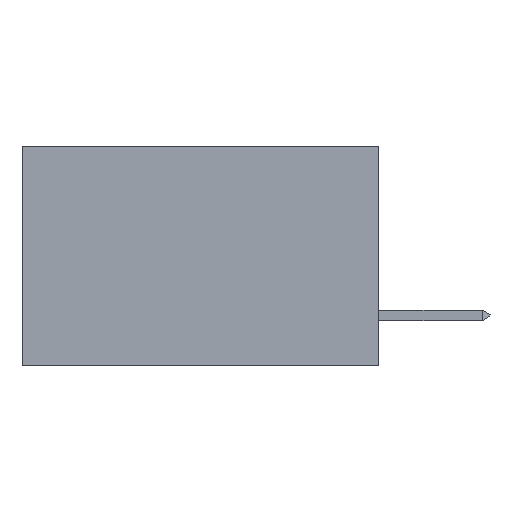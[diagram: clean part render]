
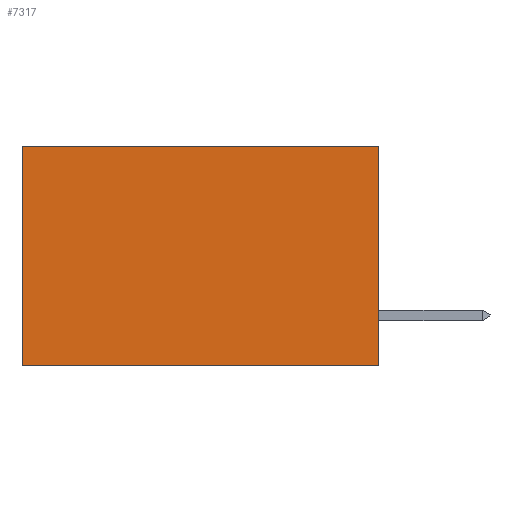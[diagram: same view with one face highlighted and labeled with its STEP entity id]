
A CAD part, left-side view. The second image highlights one B-rep face of the part: STEP entity #7317.
In plain terms, the highlighted planar face has unit normal (-1, 0, 0).
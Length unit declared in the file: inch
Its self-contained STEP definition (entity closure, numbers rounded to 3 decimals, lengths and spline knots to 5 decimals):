
#1004 = EDGE_CURVE ( 'NONE', #13466, #10811, #15204, .T. ) ;
#1601 = ORIENTED_EDGE ( 'NONE', *, *, #4666, .F. ) ;
#1602 = LINE ( 'NONE', #13977, #9259 ) ;
#2469 = LINE ( 'NONE', #5421, #9478 ) ;
#2508 = CARTESIAN_POINT ( 'NONE',  ( 0.298, 0.6, 0. ) ) ;
#3609 = PLANE ( 'NONE',  #8232 ) ;
#3677 = DIRECTION ( 'NONE',  ( 1., 0., 0. ) ) ;
#4666 = EDGE_CURVE ( 'NONE', #5327, #4895, #8896, .T. ) ;
#4877 = VECTOR ( 'NONE', #11938, 39.37008 ) ;
#4895 = VERTEX_POINT ( 'NONE', #14901 ) ;
#5012 = CARTESIAN_POINT ( 'NONE',  ( 0.298, 0., 0. ) ) ;
#5327 = VERTEX_POINT ( 'NONE', #17194 ) ;
#5421 = CARTESIAN_POINT ( 'NONE',  ( 0.298, 0., -0.37 ) ) ;
#7317 = ADVANCED_FACE ( 'NONE', ( #16875 ), #3609, .F. ) ;
#7479 = CARTESIAN_POINT ( 'NONE',  ( 0.298, 0.6, 0. ) ) ;
#7665 = ORIENTED_EDGE ( 'NONE', *, *, #1004, .T. ) ;
#8232 = AXIS2_PLACEMENT_3D ( 'NONE', #5012, #3677, #10744 ) ;
#8896 = LINE ( 'NONE', #17349, #15725 ) ;
#9259 = VECTOR ( 'NONE', #14043, 39.37008 ) ;
#9478 = VECTOR ( 'NONE', #9681, 39.37008 ) ;
#9681 = DIRECTION ( 'NONE',  ( 0., 1., 0. ) ) ;
#10510 = EDGE_LOOP ( 'NONE', ( #7665, #15460, #1601, #10550 ) ) ;
#10511 = DIRECTION ( 'NONE',  ( 0., 0., -1. ) ) ;
#10550 = ORIENTED_EDGE ( 'NONE', *, *, #10911, .T. ) ;
#10744 = DIRECTION ( 'NONE',  ( 0., 0., -1. ) ) ;
#10811 = VERTEX_POINT ( 'NONE', #13870 ) ;
#10911 = EDGE_CURVE ( 'NONE', #5327, #13466, #1602, .T. ) ;
#11938 = DIRECTION ( 'NONE',  ( 0., 0., -1. ) ) ;
#12427 = EDGE_CURVE ( 'NONE', #4895, #10811, #2469, .T. ) ;
#13466 = VERTEX_POINT ( 'NONE', #2508 ) ;
#13870 = CARTESIAN_POINT ( 'NONE',  ( 0.298, 0.6, -0.37 ) ) ;
#13977 = CARTESIAN_POINT ( 'NONE',  ( 0.298, 0., 0. ) ) ;
#14043 = DIRECTION ( 'NONE',  ( 0., 1., 0. ) ) ;
#14901 = CARTESIAN_POINT ( 'NONE',  ( 0.298, 0., -0.37 ) ) ;
#15204 = LINE ( 'NONE', #7479, #4877 ) ;
#15460 = ORIENTED_EDGE ( 'NONE', *, *, #12427, .F. ) ;
#15725 = VECTOR ( 'NONE', #10511, 39.37008 ) ;
#16875 = FACE_OUTER_BOUND ( 'NONE', #10510, .T. ) ;
#17194 = CARTESIAN_POINT ( 'NONE',  ( 0.298, 0., 0. ) ) ;
#17349 = CARTESIAN_POINT ( 'NONE',  ( 0.298, 0., 0. ) ) ;
